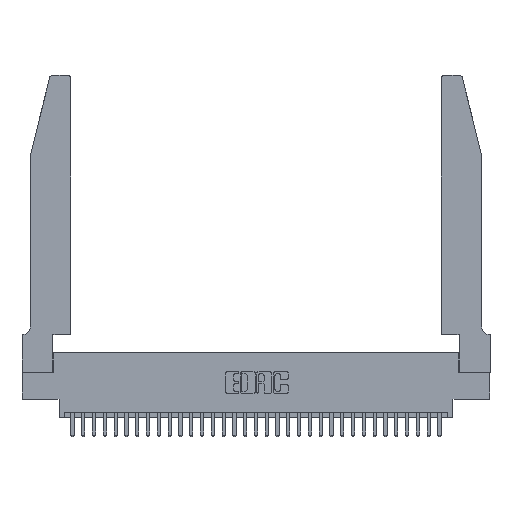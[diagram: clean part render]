
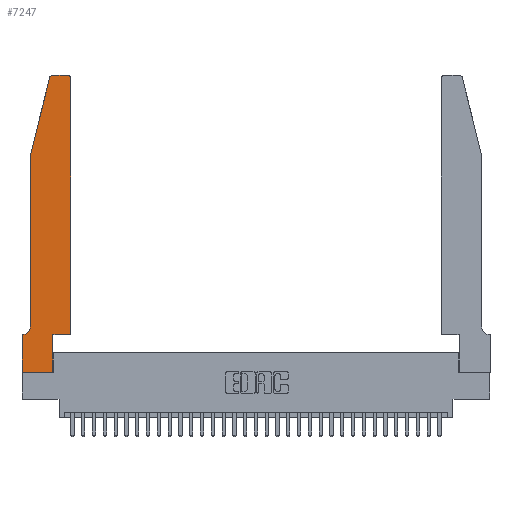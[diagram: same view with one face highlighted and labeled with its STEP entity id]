
A CAD part, top view. The second image highlights one B-rep face of the part: STEP entity #7247.
In plain terms, the highlighted planar face has unit normal (0, 0, 1).
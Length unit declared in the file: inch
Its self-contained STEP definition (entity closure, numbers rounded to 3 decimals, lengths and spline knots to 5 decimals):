
#64 = AXIS2_PLACEMENT_3D ( 'NONE', #4735, #22790, #7351 ) ;
#592 = VECTOR ( 'NONE', #18552, 39.37008 ) ;
#627 = ORIENTED_EDGE ( 'NONE', *, *, #20845, .T. ) ;
#933 = AXIS2_PLACEMENT_3D ( 'NONE', #13175, #20941, #5447 ) ;
#1394 = CARTESIAN_POINT ( 'NONE',  ( 0.2605, 2.75, 0.37 ) ) ;
#2074 = VERTEX_POINT ( 'NONE', #26087 ) ;
#2334 = VERTEX_POINT ( 'NONE', #21861 ) ;
#2437 = CARTESIAN_POINT ( 'NONE',  ( 0.4205, 2.72, 0.37 ) ) ;
#2933 = EDGE_CURVE ( 'NONE', #6012, #10517, #20488, .T. ) ;
#3978 = DIRECTION ( 'NONE',  ( -1., 0., 0. ) ) ;
#3991 = DIRECTION ( 'NONE',  ( -1., 0., 0. ) ) ;
#4735 = CARTESIAN_POINT ( 'NONE',  ( 0.284, 2.72, 0.37 ) ) ;
#4818 = VERTEX_POINT ( 'NONE', #21644 ) ;
#4859 = CARTESIAN_POINT ( 'NONE',  ( 0.25487, 2.72718, 0.37 ) ) ;
#4976 = CARTESIAN_POINT ( 'NONE',  ( 0.2865, 0., 0.37 ) ) ;
#5045 = EDGE_CURVE ( 'NONE', #12075, #6012, #21552, .T. ) ;
#5060 = DIRECTION ( 'NONE',  ( 1., 0., 0. ) ) ;
#5229 = VERTEX_POINT ( 'NONE', #26166 ) ;
#5231 = PLANE ( 'NONE',  #933 ) ;
#5280 = ORIENTED_EDGE ( 'NONE', *, *, #17224, .T. ) ;
#5402 = EDGE_CURVE ( 'NONE', #10555, #12075, #12326, .T. ) ;
#5447 = DIRECTION ( 'NONE',  ( 1., 0., 0. ) ) ;
#5479 = CARTESIAN_POINT ( 'NONE',  ( 0., 0.35, 0.37 ) ) ;
#6012 = VERTEX_POINT ( 'NONE', #14158 ) ;
#6788 = VERTEX_POINT ( 'NONE', #32644 ) ;
#6819 = CIRCLE ( 'NONE', #12155, 0.03 ) ;
#7247 = ADVANCED_FACE ( 'NONE', ( #31910 ), #5231, .T. ) ;
#7351 = DIRECTION ( 'NONE',  ( 1., 0., 0. ) ) ;
#7537 = CARTESIAN_POINT ( 'NONE',  ( 0.2865, 0.35, 0.37 ) ) ;
#7634 = ORIENTED_EDGE ( 'NONE', *, *, #15418, .T. ) ;
#8668 = VERTEX_POINT ( 'NONE', #5479 ) ;
#9131 = VECTOR ( 'NONE', #3978, 39.37008 ) ;
#9344 = VECTOR ( 'NONE', #26290, 39.37008 ) ;
#10098 = DIRECTION ( 'NONE',  ( 0., 0., -1. ) ) ;
#10517 = VERTEX_POINT ( 'NONE', #27356 ) ;
#10555 = VERTEX_POINT ( 'NONE', #19869 ) ;
#12075 = VERTEX_POINT ( 'NONE', #4976 ) ;
#12138 = VECTOR ( 'NONE', #25167, 39.37008 ) ;
#12155 = AXIS2_PLACEMENT_3D ( 'NONE', #2437, #20543, #5060 ) ;
#12198 = EDGE_CURVE ( 'NONE', #8668, #10555, #21224, .T. ) ;
#12326 = LINE ( 'NONE', #31955, #30423 ) ;
#12928 = ORIENTED_EDGE ( 'NONE', *, *, #30896, .T. ) ;
#13079 = VERTEX_POINT ( 'NONE', #23914 ) ;
#13175 = CARTESIAN_POINT ( 'NONE',  ( 0., 0.35, 0.37 ) ) ;
#13256 = ORIENTED_EDGE ( 'NONE', *, *, #2933, .T. ) ;
#14083 = CARTESIAN_POINT ( 'NONE',  ( 0.4505, 0.35, 0.37 ) ) ;
#14115 = CIRCLE ( 'NONE', #64, 0.03 ) ;
#14158 = CARTESIAN_POINT ( 'NONE',  ( 0.2865, 0.35, 0.37 ) ) ;
#14744 = EDGE_CURVE ( 'NONE', #2074, #13079, #20218, .T. ) ;
#15418 = EDGE_CURVE ( 'NONE', #6788, #2334, #6819, .T. ) ;
#15944 = CARTESIAN_POINT ( 'NONE',  ( 0., 0., 0.37 ) ) ;
#16215 = LINE ( 'NONE', #18608, #9344 ) ;
#16349 = VERTEX_POINT ( 'NONE', #4859 ) ;
#16722 = VECTOR ( 'NONE', #3991, 39.37008 ) ;
#16893 = AXIS2_PLACEMENT_3D ( 'NONE', #25477, #10098, #28081 ) ;
#17224 = EDGE_CURVE ( 'NONE', #10517, #6788, #17529, .T. ) ;
#17529 = LINE ( 'NONE', #18612, #30395 ) ;
#17539 = LINE ( 'NONE', #1394, #16722 ) ;
#18552 = DIRECTION ( 'NONE',  ( 0., -1., 0. ) ) ;
#18608 = CARTESIAN_POINT ( 'NONE',  ( 0.0755, 2., 0.37 ) ) ;
#18612 = CARTESIAN_POINT ( 'NONE',  ( 0.4505, 0.35, 0.37 ) ) ;
#19266 = DIRECTION ( 'NONE',  ( 1., 0., 0. ) ) ;
#19537 = ORIENTED_EDGE ( 'NONE', *, *, #5045, .T. ) ;
#19869 = CARTESIAN_POINT ( 'NONE',  ( 0., 0., 0.37 ) ) ;
#20218 = CIRCLE ( 'NONE', #16893, 0.07 ) ;
#20223 = EDGE_CURVE ( 'NONE', #4818, #2074, #24969, .T. ) ;
#20488 = LINE ( 'NONE', #14083, #33354 ) ;
#20543 = DIRECTION ( 'NONE',  ( 0., 0., 1. ) ) ;
#20747 = VECTOR ( 'NONE', #25521, 39.37008 ) ;
#20825 = ORIENTED_EDGE ( 'NONE', *, *, #5402, .T. ) ;
#20845 = EDGE_CURVE ( 'NONE', #5229, #16349, #14115, .T. ) ;
#20941 = DIRECTION ( 'NONE',  ( 0., 0., 1. ) ) ;
#21193 = DIRECTION ( 'NONE',  ( 0., 1., 0. ) ) ;
#21224 = LINE ( 'NONE', #15944, #592 ) ;
#21495 = ORIENTED_EDGE ( 'NONE', *, *, #12198, .T. ) ;
#21552 = LINE ( 'NONE', #7537, #20747 ) ;
#21644 = CARTESIAN_POINT ( 'NONE',  ( 0.0755, 2., 0.37 ) ) ;
#21861 = CARTESIAN_POINT ( 'NONE',  ( 0.4205, 2.75, 0.37 ) ) ;
#22790 = DIRECTION ( 'NONE',  ( 0., 0., 1. ) ) ;
#23070 = EDGE_LOOP ( 'NONE', ( #12928, #627, #26878, #23164, #28700, #31629, #21495, #20825, #19537, #13256, #5280, #7634 ) ) ;
#23164 = ORIENTED_EDGE ( 'NONE', *, *, #20223, .T. ) ;
#23914 = CARTESIAN_POINT ( 'NONE',  ( 0.0055, 0.35, 0.37 ) ) ;
#24182 = DIRECTION ( 'NONE',  ( 1., 0., 0. ) ) ;
#24606 = CARTESIAN_POINT ( 'NONE',  ( 0.0755, 0.35, 0.37 ) ) ;
#24969 = LINE ( 'NONE', #32960, #12138 ) ;
#25167 = DIRECTION ( 'NONE',  ( 0., -1., 0. ) ) ;
#25477 = CARTESIAN_POINT ( 'NONE',  ( 0.0055, 0.42, 0.37 ) ) ;
#25521 = DIRECTION ( 'NONE',  ( 0., 1., 0. ) ) ;
#26087 = CARTESIAN_POINT ( 'NONE',  ( 0.0755, 0.42, 0.37 ) ) ;
#26166 = CARTESIAN_POINT ( 'NONE',  ( 0.284, 2.75, 0.37 ) ) ;
#26180 = EDGE_CURVE ( 'NONE', #16349, #4818, #16215, .T. ) ;
#26290 = DIRECTION ( 'NONE',  ( -0.239, -0.971, 0. ) ) ;
#26878 = ORIENTED_EDGE ( 'NONE', *, *, #26180, .T. ) ;
#27356 = CARTESIAN_POINT ( 'NONE',  ( 0.4505, 0.35, 0.37 ) ) ;
#28081 = DIRECTION ( 'NONE',  ( -1., 0., 0. ) ) ;
#28700 = ORIENTED_EDGE ( 'NONE', *, *, #14744, .T. ) ;
#28823 = EDGE_CURVE ( 'NONE', #13079, #8668, #29692, .T. ) ;
#29692 = LINE ( 'NONE', #24606, #9131 ) ;
#30395 = VECTOR ( 'NONE', #21193, 39.37008 ) ;
#30423 = VECTOR ( 'NONE', #24182, 39.37008 ) ;
#30896 = EDGE_CURVE ( 'NONE', #2334, #5229, #17539, .T. ) ;
#31629 = ORIENTED_EDGE ( 'NONE', *, *, #28823, .T. ) ;
#31910 = FACE_OUTER_BOUND ( 'NONE', #23070, .T. ) ;
#31955 = CARTESIAN_POINT ( 'NONE',  ( 0., 0., 0.37 ) ) ;
#32644 = CARTESIAN_POINT ( 'NONE',  ( 0.4505, 2.72, 0.37 ) ) ;
#32960 = CARTESIAN_POINT ( 'NONE',  ( 0.0755, 2., 0.37 ) ) ;
#33354 = VECTOR ( 'NONE', #19266, 39.37008 ) ;
